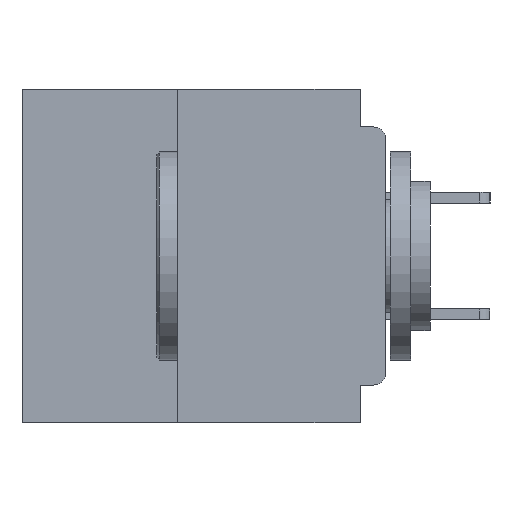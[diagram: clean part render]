
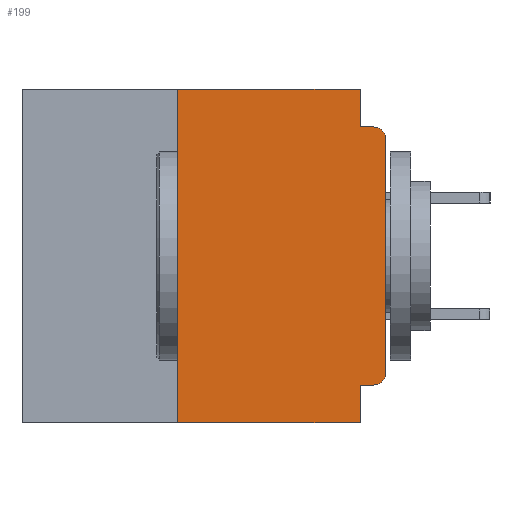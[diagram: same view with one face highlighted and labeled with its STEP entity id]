
A CAD part, left-side view. The second image highlights one B-rep face of the part: STEP entity #199.
In plain terms, the highlighted planar face has unit normal (-1, 0, 0).
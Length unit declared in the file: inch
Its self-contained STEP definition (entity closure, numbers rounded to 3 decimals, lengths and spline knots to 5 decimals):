
#199 = ADVANCED_FACE ( 'NONE', ( #1658 ), #21610, .F. ) ;
#494 = VECTOR ( 'NONE', #21043, 39.37008 ) ;
#585 = EDGE_CURVE ( 'NONE', #6946, #18425, #12876, .T. ) ;
#959 = VECTOR ( 'NONE', #5807, 39.37008 ) ;
#1256 = CARTESIAN_POINT ( 'NONE',  ( 0., 0.25, 0. ) ) ;
#1658 = FACE_OUTER_BOUND ( 'NONE', #15624, .T. ) ;
#2336 = VECTOR ( 'NONE', #35503, 39.37008 ) ;
#2393 = ORIENTED_EDGE ( 'NONE', *, *, #32781, .F. ) ;
#2844 = LINE ( 'NONE', #12007, #30204 ) ;
#3387 = AXIS2_PLACEMENT_3D ( 'NONE', #38694, #36175, #17074 ) ;
#3775 = VECTOR ( 'NONE', #25118, 39.37008 ) ;
#4982 = ORIENTED_EDGE ( 'NONE', *, *, #36910, .T. ) ;
#5807 = DIRECTION ( 'NONE',  ( 0., 0., -1. ) ) ;
#6186 = CARTESIAN_POINT ( 'NONE',  ( 0., 0.031, -0.4 ) ) ;
#6946 = VERTEX_POINT ( 'NONE', #37439 ) ;
#7501 = CARTESIAN_POINT ( 'NONE',  ( 0., 0., -0.34 ) ) ;
#8053 = LINE ( 'NONE', #38840, #26277 ) ;
#8482 = EDGE_CURVE ( 'NONE', #43718, #16301, #41985, .T. ) ;
#8580 = DIRECTION ( 'NONE',  ( 0., -1., 0. ) ) ;
#8588 = VERTEX_POINT ( 'NONE', #27912 ) ;
#8795 = EDGE_CURVE ( 'NONE', #20916, #30513, #2844, .T. ) ;
#9230 = CARTESIAN_POINT ( 'NONE',  ( 0., 0.031, -0.045 ) ) ;
#9973 = CARTESIAN_POINT ( 'NONE',  ( 0., 0.015, -0.06 ) ) ;
#10074 = LINE ( 'NONE', #19421, #959 ) ;
#11433 = EDGE_CURVE ( 'NONE', #6946, #20916, #21893, .T. ) ;
#11920 = ORIENTED_EDGE ( 'NONE', *, *, #19914, .F. ) ;
#12007 = CARTESIAN_POINT ( 'NONE',  ( 0., 0.437, 0. ) ) ;
#12605 = CARTESIAN_POINT ( 'NONE',  ( 0., 0.031, 0. ) ) ;
#12876 = LINE ( 'NONE', #38046, #3775 ) ;
#13401 = DIRECTION ( 'NONE',  ( 0., 0., -1. ) ) ;
#14430 = ORIENTED_EDGE ( 'NONE', *, *, #35671, .F. ) ;
#14759 = ORIENTED_EDGE ( 'NONE', *, *, #8482, .F. ) ;
#15484 = VERTEX_POINT ( 'NONE', #7501 ) ;
#15624 = EDGE_LOOP ( 'NONE', ( #38857, #23894, #14430, #11920, #21304, #21971, #19394, #2393, #14759, #4982 ) ) ;
#16301 = VERTEX_POINT ( 'NONE', #39304 ) ;
#17074 = DIRECTION ( 'NONE',  ( 0., 0., -1. ) ) ;
#17107 = CARTESIAN_POINT ( 'NONE',  ( 0., 0., -0.355 ) ) ;
#18068 = DIRECTION ( 'NONE',  ( -1., 0., 0. ) ) ;
#18352 = VERTEX_POINT ( 'NONE', #9230 ) ;
#18425 = VERTEX_POINT ( 'NONE', #6186 ) ;
#19394 = ORIENTED_EDGE ( 'NONE', *, *, #585, .T. ) ;
#19421 = CARTESIAN_POINT ( 'NONE',  ( 0., 0.031, 0. ) ) ;
#19914 = EDGE_CURVE ( 'NONE', #30513, #18352, #10074, .T. ) ;
#19983 = AXIS2_PLACEMENT_3D ( 'NONE', #9973, #33915, #13401 ) ;
#20031 = CARTESIAN_POINT ( 'NONE',  ( 0., 0.25, -0.4 ) ) ;
#20553 = DIRECTION ( 'NONE',  ( 0., 1., 0. ) ) ;
#20889 = CIRCLE ( 'NONE', #19983, 0.015 ) ;
#20916 = VERTEX_POINT ( 'NONE', #1256 ) ;
#21043 = DIRECTION ( 'NONE',  ( 0., -1., 0. ) ) ;
#21304 = ORIENTED_EDGE ( 'NONE', *, *, #8795, .F. ) ;
#21610 = PLANE ( 'NONE',  #3387 ) ;
#21893 = LINE ( 'NONE', #20031, #29951 ) ;
#21971 = ORIENTED_EDGE ( 'NONE', *, *, #11433, .F. ) ;
#23894 = ORIENTED_EDGE ( 'NONE', *, *, #37282, .T. ) ;
#24690 = CIRCLE ( 'NONE', #35475, 0.015 ) ;
#25118 = DIRECTION ( 'NONE',  ( 0., -1., 0. ) ) ;
#26277 = VECTOR ( 'NONE', #31981, 39.37008 ) ;
#27912 = CARTESIAN_POINT ( 'NONE',  ( 0., 0.015, -0.045 ) ) ;
#28774 = CARTESIAN_POINT ( 'NONE',  ( 0., 0.031, -0.4 ) ) ;
#29702 = LINE ( 'NONE', #28774, #2336 ) ;
#29951 = VECTOR ( 'NONE', #40555, 39.37008 ) ;
#30204 = VECTOR ( 'NONE', #8580, 39.37008 ) ;
#30513 = VERTEX_POINT ( 'NONE', #12605 ) ;
#30943 = CARTESIAN_POINT ( 'NONE',  ( 0., 0.015, -0.355 ) ) ;
#31506 = VERTEX_POINT ( 'NONE', #38591 ) ;
#31981 = DIRECTION ( 'NONE',  ( 0., 0., 1. ) ) ;
#32781 = EDGE_CURVE ( 'NONE', #16301, #18425, #29702, .T. ) ;
#32904 = VECTOR ( 'NONE', #20553, 39.37008 ) ;
#33915 = DIRECTION ( 'NONE',  ( -1., 0., 0. ) ) ;
#34673 = CARTESIAN_POINT ( 'NONE',  ( 0., 0., -0.045 ) ) ;
#35475 = AXIS2_PLACEMENT_3D ( 'NONE', #38601, #18068, #42023 ) ;
#35503 = DIRECTION ( 'NONE',  ( 0., 0., -1. ) ) ;
#35671 = EDGE_CURVE ( 'NONE', #18352, #8588, #37988, .T. ) ;
#36175 = DIRECTION ( 'NONE',  ( 1., 0., 0. ) ) ;
#36910 = EDGE_CURVE ( 'NONE', #43718, #15484, #24690, .T. ) ;
#37282 = EDGE_CURVE ( 'NONE', #31506, #8588, #20889, .T. ) ;
#37439 = CARTESIAN_POINT ( 'NONE',  ( 0., 0.25, -0.4 ) ) ;
#37988 = LINE ( 'NONE', #34673, #494 ) ;
#38046 = CARTESIAN_POINT ( 'NONE',  ( 0., 0.437, -0.4 ) ) ;
#38591 = CARTESIAN_POINT ( 'NONE',  ( 0., 0., -0.06 ) ) ;
#38601 = CARTESIAN_POINT ( 'NONE',  ( 0., 0.015, -0.34 ) ) ;
#38694 = CARTESIAN_POINT ( 'NONE',  ( 0., 0.437, 0. ) ) ;
#38840 = CARTESIAN_POINT ( 'NONE',  ( 0., 0., 0. ) ) ;
#38857 = ORIENTED_EDGE ( 'NONE', *, *, #43957, .T. ) ;
#39304 = CARTESIAN_POINT ( 'NONE',  ( 0., 0.031, -0.355 ) ) ;
#40555 = DIRECTION ( 'NONE',  ( 0., 0., 1. ) ) ;
#41985 = LINE ( 'NONE', #17107, #32904 ) ;
#42023 = DIRECTION ( 'NONE',  ( 0., 0., -1. ) ) ;
#43718 = VERTEX_POINT ( 'NONE', #30943 ) ;
#43957 = EDGE_CURVE ( 'NONE', #15484, #31506, #8053, .T. ) ;
